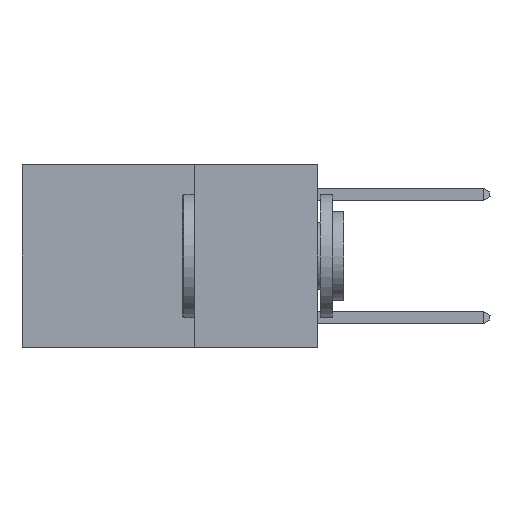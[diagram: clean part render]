
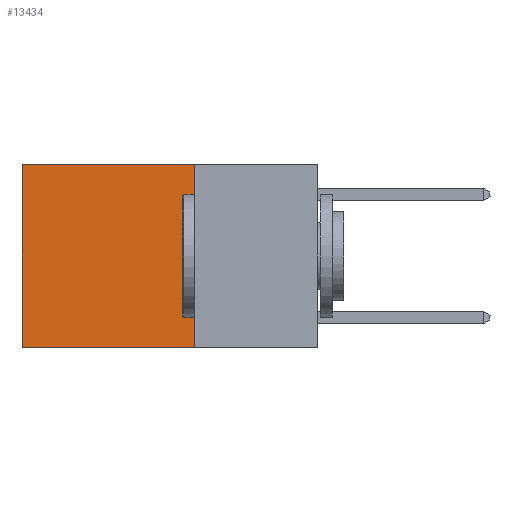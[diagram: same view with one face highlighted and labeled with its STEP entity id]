
A CAD part, left-side view. The second image highlights one B-rep face of the part: STEP entity #13434.
In plain terms, the highlighted planar face has unit normal (-1, 0, 0).
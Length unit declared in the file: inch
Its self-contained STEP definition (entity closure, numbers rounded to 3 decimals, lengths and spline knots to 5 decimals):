
#701 = EDGE_CURVE ( 'NONE', #3364, #10156, #16183, .T. ) ;
#755 = FACE_OUTER_BOUND ( 'NONE', #15100, .T. ) ;
#954 = CARTESIAN_POINT ( 'NONE',  ( 0.2625, 0.25, -0.37 ) ) ;
#1672 = VERTEX_POINT ( 'NONE', #14352 ) ;
#1754 = LINE ( 'NONE', #4579, #8274 ) ;
#1827 = DIRECTION ( 'NONE',  ( 0., 0., -1. ) ) ;
#3119 = DIRECTION ( 'NONE',  ( 0., 1., 0. ) ) ;
#3364 = VERTEX_POINT ( 'NONE', #10916 ) ;
#4384 = CARTESIAN_POINT ( 'NONE',  ( 0.2625, 0.25, 0. ) ) ;
#4527 = EDGE_CURVE ( 'NONE', #12900, #3364, #1754, .T. ) ;
#4579 = CARTESIAN_POINT ( 'NONE',  ( 0.2625, 0.25, 0. ) ) ;
#4853 = DIRECTION ( 'NONE',  ( 0., 0., -1. ) ) ;
#4921 = DIRECTION ( 'NONE',  ( 0., 1., 0. ) ) ;
#4949 = EDGE_CURVE ( 'NONE', #12900, #1672, #6467, .T. ) ;
#5437 = CARTESIAN_POINT ( 'NONE',  ( 0.2625, 0.6, -0.37 ) ) ;
#5622 = PLANE ( 'NONE',  #12005 ) ;
#6098 = CARTESIAN_POINT ( 'NONE',  ( 0.2625, 0.6, 0. ) ) ;
#6467 = LINE ( 'NONE', #4384, #12612 ) ;
#8225 = CARTESIAN_POINT ( 'NONE',  ( 0.2625, 0.25, 0. ) ) ;
#8274 = VECTOR ( 'NONE', #3119, 39.37008 ) ;
#9966 = ORIENTED_EDGE ( 'NONE', *, *, #15870, .F. ) ;
#10156 = VERTEX_POINT ( 'NONE', #5437 ) ;
#10916 = CARTESIAN_POINT ( 'NONE',  ( 0.2625, 0.6, 0. ) ) ;
#12005 = AXIS2_PLACEMENT_3D ( 'NONE', #8225, #13360, #1827 ) ;
#12264 = ORIENTED_EDGE ( 'NONE', *, *, #701, .T. ) ;
#12612 = VECTOR ( 'NONE', #13206, 39.37008 ) ;
#12900 = VERTEX_POINT ( 'NONE', #14896 ) ;
#13206 = DIRECTION ( 'NONE',  ( 0., 0., -1. ) ) ;
#13360 = DIRECTION ( 'NONE',  ( 1., 0., 0. ) ) ;
#13434 = ADVANCED_FACE ( 'NONE', ( #755 ), #5622, .F. ) ;
#13971 = LINE ( 'NONE', #954, #16584 ) ;
#14352 = CARTESIAN_POINT ( 'NONE',  ( 0.2625, 0.25, -0.37 ) ) ;
#14896 = CARTESIAN_POINT ( 'NONE',  ( 0.2625, 0.25, 0. ) ) ;
#15084 = ORIENTED_EDGE ( 'NONE', *, *, #4949, .F. ) ;
#15100 = EDGE_LOOP ( 'NONE', ( #12264, #9966, #15084, #15390 ) ) ;
#15390 = ORIENTED_EDGE ( 'NONE', *, *, #4527, .T. ) ;
#15870 = EDGE_CURVE ( 'NONE', #1672, #10156, #13971, .T. ) ;
#15903 = VECTOR ( 'NONE', #4853, 39.37008 ) ;
#16183 = LINE ( 'NONE', #6098, #15903 ) ;
#16584 = VECTOR ( 'NONE', #4921, 39.37008 ) ;
